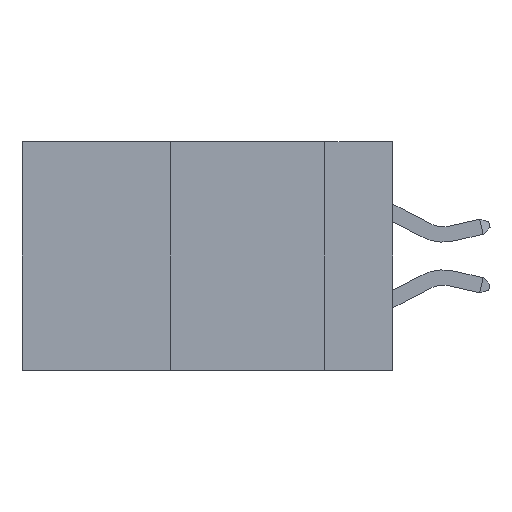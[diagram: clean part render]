
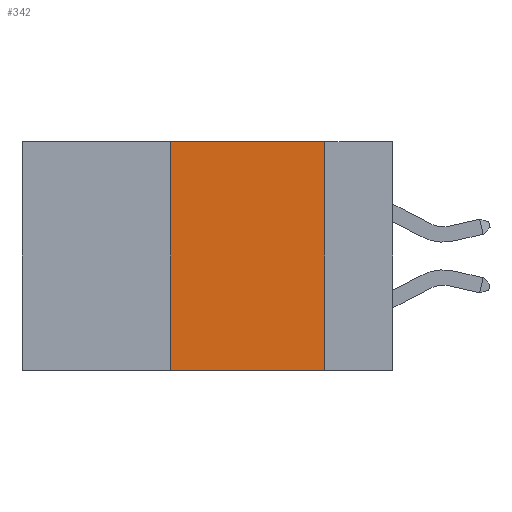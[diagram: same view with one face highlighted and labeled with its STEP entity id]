
A CAD part, left-side view. The second image highlights one B-rep face of the part: STEP entity #342.
In plain terms, the highlighted planar face has unit normal (-1, 0, 0).
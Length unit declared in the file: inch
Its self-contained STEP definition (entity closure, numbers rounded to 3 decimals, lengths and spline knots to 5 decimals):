
#342 = ADVANCED_FACE ( 'NONE', ( #11442 ), #19375, .F. ) ;
#435 = EDGE_CURVE ( 'NONE', #9299, #3156, #22047, .T. ) ;
#1763 = CARTESIAN_POINT ( 'NONE',  ( 0., 0.36, -0.37 ) ) ;
#1907 = CARTESIAN_POINT ( 'NONE',  ( 0., 0.6, -0.37 ) ) ;
#3156 = VERTEX_POINT ( 'NONE', #9319 ) ;
#3224 = ORIENTED_EDGE ( 'NONE', *, *, #5519, .F. ) ;
#3611 = CARTESIAN_POINT ( 'NONE',  ( 0., 0.11, 0. ) ) ;
#4195 = VECTOR ( 'NONE', #19958, 39.37008 ) ;
#5519 = EDGE_CURVE ( 'NONE', #21172, #9299, #7520, .T. ) ;
#5587 = ORIENTED_EDGE ( 'NONE', *, *, #435, .F. ) ;
#5704 = VECTOR ( 'NONE', #22452, 39.37008 ) ;
#6217 = CARTESIAN_POINT ( 'NONE',  ( 0., 0.6, 0. ) ) ;
#7071 = EDGE_CURVE ( 'NONE', #21172, #7083, #10504, .T. ) ;
#7083 = VERTEX_POINT ( 'NONE', #20764 ) ;
#7520 = LINE ( 'NONE', #14469, #9228 ) ;
#7535 = EDGE_LOOP ( 'NONE', ( #20955, #5587, #3224, #8000 ) ) ;
#8000 = ORIENTED_EDGE ( 'NONE', *, *, #7071, .T. ) ;
#8161 = LINE ( 'NONE', #3611, #4195 ) ;
#8806 = DIRECTION ( 'NONE',  ( 1., 0., 0. ) ) ;
#9070 = DIRECTION ( 'NONE',  ( 0., 0., 1. ) ) ;
#9228 = VECTOR ( 'NONE', #9070, 39.37008 ) ;
#9299 = VERTEX_POINT ( 'NONE', #20551 ) ;
#9319 = CARTESIAN_POINT ( 'NONE',  ( 0., 0.11, 0. ) ) ;
#9564 = EDGE_CURVE ( 'NONE', #3156, #7083, #8161, .T. ) ;
#10504 = LINE ( 'NONE', #1907, #5704 ) ;
#10597 = AXIS2_PLACEMENT_3D ( 'NONE', #17875, #8806, #12267 ) ;
#11182 = VECTOR ( 'NONE', #22464, 39.37008 ) ;
#11442 = FACE_OUTER_BOUND ( 'NONE', #7535, .T. ) ;
#12267 = DIRECTION ( 'NONE',  ( 0., 0., -1. ) ) ;
#14469 = CARTESIAN_POINT ( 'NONE',  ( 0., 0.36, 0. ) ) ;
#17875 = CARTESIAN_POINT ( 'NONE',  ( 0., 0.6, 0. ) ) ;
#19375 = PLANE ( 'NONE',  #10597 ) ;
#19958 = DIRECTION ( 'NONE',  ( 0., 0., -1. ) ) ;
#20551 = CARTESIAN_POINT ( 'NONE',  ( 0., 0.36, 0. ) ) ;
#20764 = CARTESIAN_POINT ( 'NONE',  ( 0., 0.11, -0.37 ) ) ;
#20955 = ORIENTED_EDGE ( 'NONE', *, *, #9564, .F. ) ;
#21172 = VERTEX_POINT ( 'NONE', #1763 ) ;
#22047 = LINE ( 'NONE', #6217, #11182 ) ;
#22452 = DIRECTION ( 'NONE',  ( 0., -1., 0. ) ) ;
#22464 = DIRECTION ( 'NONE',  ( 0., -1., 0. ) ) ;
